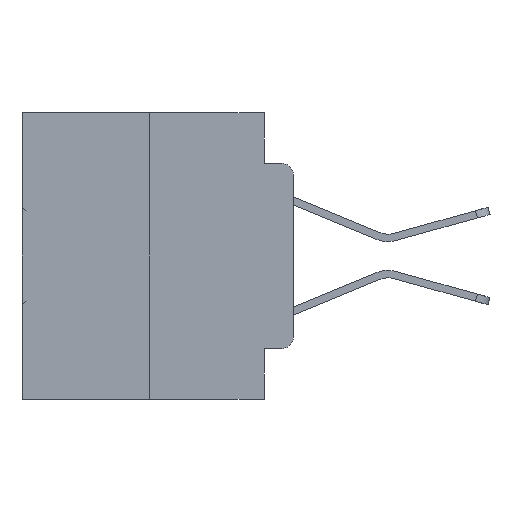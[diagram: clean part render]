
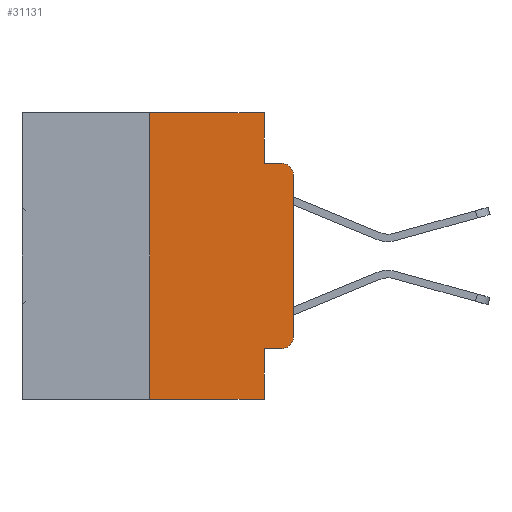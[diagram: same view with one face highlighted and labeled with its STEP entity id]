
A CAD part, left-side view. The second image highlights one B-rep face of the part: STEP entity #31131.
In plain terms, the highlighted planar face has unit normal (-1, 0, 0).
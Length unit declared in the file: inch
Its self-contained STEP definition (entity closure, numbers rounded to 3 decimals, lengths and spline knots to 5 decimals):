
#1025 = ORIENTED_EDGE ( 'NONE', *, *, #8516, .F. ) ;
#1238 = VERTEX_POINT ( 'NONE', #7258 ) ;
#1421 = ORIENTED_EDGE ( 'NONE', *, *, #26713, .T. ) ;
#1630 = EDGE_CURVE ( 'NONE', #18793, #30421, #24792, .T. ) ;
#1648 = VERTEX_POINT ( 'NONE', #25018 ) ;
#1846 = ORIENTED_EDGE ( 'NONE', *, *, #18257, .T. ) ;
#1852 = CARTESIAN_POINT ( 'NONE',  ( 0., 0.473, -0.5 ) ) ;
#3030 = ORIENTED_EDGE ( 'NONE', *, *, #29898, .F. ) ;
#3346 = EDGE_CURVE ( 'NONE', #16393, #30421, #4050, .T. ) ;
#3467 = DIRECTION ( 'NONE',  ( 0., 0., 1. ) ) ;
#3589 = CARTESIAN_POINT ( 'NONE',  ( 0., 0.051, -0.4115 ) ) ;
#3767 = VECTOR ( 'NONE', #28700, 39.37008 ) ;
#3779 = CARTESIAN_POINT ( 'NONE',  ( 0., 0.25, -0.5 ) ) ;
#4050 = LINE ( 'NONE', #28193, #22817 ) ;
#4171 = CARTESIAN_POINT ( 'NONE',  ( 0., 0.473, 0. ) ) ;
#4619 = VERTEX_POINT ( 'NONE', #8274 ) ;
#4640 = ORIENTED_EDGE ( 'NONE', *, *, #25094, .F. ) ;
#4883 = AXIS2_PLACEMENT_3D ( 'NONE', #17236, #7419, #24492 ) ;
#4959 = PLANE ( 'NONE',  #4883 ) ;
#5057 = LINE ( 'NONE', #21736, #17384 ) ;
#5177 = DIRECTION ( 'NONE',  ( 0., 0., -1. ) ) ;
#5920 = LINE ( 'NONE', #28124, #19065 ) ;
#7258 = CARTESIAN_POINT ( 'NONE',  ( 0., 0., -0.3915 ) ) ;
#7419 = DIRECTION ( 'NONE',  ( 1., 0., 0. ) ) ;
#7840 = LINE ( 'NONE', #20682, #15943 ) ;
#8078 = ORIENTED_EDGE ( 'NONE', *, *, #1630, .T. ) ;
#8274 = CARTESIAN_POINT ( 'NONE',  ( 0., 0.02, -0.4115 ) ) ;
#8516 = EDGE_CURVE ( 'NONE', #19788, #1648, #23984, .T. ) ;
#9701 = EDGE_LOOP ( 'NONE', ( #1421, #8078, #21119, #3030, #16188, #4640, #12731, #1025, #14278, #1846 ) ) ;
#9738 = CARTESIAN_POINT ( 'NONE',  ( 0., 0.051, -0.4115 ) ) ;
#10008 = CIRCLE ( 'NONE', #16569, 0.02 ) ;
#11039 = VECTOR ( 'NONE', #5177, 39.37008 ) ;
#11698 = AXIS2_PLACEMENT_3D ( 'NONE', #22172, #13034, #18883 ) ;
#12731 = ORIENTED_EDGE ( 'NONE', *, *, #18904, .T. ) ;
#13034 = DIRECTION ( 'NONE',  ( -1., 0., 0. ) ) ;
#13632 = DIRECTION ( 'NONE',  ( 0., 0., -1. ) ) ;
#13913 = CARTESIAN_POINT ( 'NONE',  ( 0., 0., -0.1085 ) ) ;
#14278 = ORIENTED_EDGE ( 'NONE', *, *, #18343, .T. ) ;
#14365 = CARTESIAN_POINT ( 'NONE',  ( 0., 0.051, -0.0885 ) ) ;
#14369 = DIRECTION ( 'NONE',  ( -1., 0., 0. ) ) ;
#15943 = VECTOR ( 'NONE', #3467, 39.37008 ) ;
#16188 = ORIENTED_EDGE ( 'NONE', *, *, #26628, .F. ) ;
#16339 = VERTEX_POINT ( 'NONE', #28628 ) ;
#16393 = VERTEX_POINT ( 'NONE', #14365 ) ;
#16569 = AXIS2_PLACEMENT_3D ( 'NONE', #28843, #14369, #31193 ) ;
#17058 = DIRECTION ( 'NONE',  ( 0., -1., 0. ) ) ;
#17236 = CARTESIAN_POINT ( 'NONE',  ( 0., 0.473, 0. ) ) ;
#17384 = VECTOR ( 'NONE', #24153, 39.37008 ) ;
#18257 = EDGE_CURVE ( 'NONE', #4619, #1238, #10008, .T. ) ;
#18343 = EDGE_CURVE ( 'NONE', #19788, #4619, #26346, .T. ) ;
#18793 = VERTEX_POINT ( 'NONE', #13913 ) ;
#18883 = DIRECTION ( 'NONE',  ( 0., 0., -1. ) ) ;
#18904 = EDGE_CURVE ( 'NONE', #27709, #1648, #29679, .T. ) ;
#19065 = VECTOR ( 'NONE', #13632, 39.37008 ) ;
#19788 = VERTEX_POINT ( 'NONE', #3589 ) ;
#19915 = CARTESIAN_POINT ( 'NONE',  ( 0., 0.051, 0. ) ) ;
#20430 = LINE ( 'NONE', #4171, #26042 ) ;
#20534 = CARTESIAN_POINT ( 'NONE',  ( 0., 0.02, -0.0885 ) ) ;
#20682 = CARTESIAN_POINT ( 'NONE',  ( 0., 0.25, 0. ) ) ;
#21119 = ORIENTED_EDGE ( 'NONE', *, *, #3346, .F. ) ;
#21420 = DIRECTION ( 'NONE',  ( 0., -1., 0. ) ) ;
#21736 = CARTESIAN_POINT ( 'NONE',  ( 0., 0., 0. ) ) ;
#22172 = CARTESIAN_POINT ( 'NONE',  ( 0., 0.02, -0.1085 ) ) ;
#22331 = DIRECTION ( 'NONE',  ( 0., -1., 0. ) ) ;
#22817 = VECTOR ( 'NONE', #22331, 39.37008 ) ;
#23984 = LINE ( 'NONE', #19915, #11039 ) ;
#24153 = DIRECTION ( 'NONE',  ( 0., 0., 1. ) ) ;
#24492 = DIRECTION ( 'NONE',  ( 0., 0., -1. ) ) ;
#24792 = CIRCLE ( 'NONE', #11698, 0.02 ) ;
#25018 = CARTESIAN_POINT ( 'NONE',  ( 0., 0.051, -0.5 ) ) ;
#25094 = EDGE_CURVE ( 'NONE', #27709, #31348, #7840, .T. ) ;
#25593 = VECTOR ( 'NONE', #17058, 39.37008 ) ;
#25751 = FACE_OUTER_BOUND ( 'NONE', #9701, .T. ) ;
#26042 = VECTOR ( 'NONE', #21420, 39.37008 ) ;
#26346 = LINE ( 'NONE', #9738, #25593 ) ;
#26628 = EDGE_CURVE ( 'NONE', #31348, #16339, #20430, .T. ) ;
#26713 = EDGE_CURVE ( 'NONE', #1238, #18793, #5057, .T. ) ;
#27709 = VERTEX_POINT ( 'NONE', #3779 ) ;
#28124 = CARTESIAN_POINT ( 'NONE',  ( 0., 0.051, 0. ) ) ;
#28193 = CARTESIAN_POINT ( 'NONE',  ( 0., 0.051, -0.0885 ) ) ;
#28628 = CARTESIAN_POINT ( 'NONE',  ( 0., 0.051, 0. ) ) ;
#28700 = DIRECTION ( 'NONE',  ( 0., -1., 0. ) ) ;
#28843 = CARTESIAN_POINT ( 'NONE',  ( 0., 0.02, -0.3915 ) ) ;
#29679 = LINE ( 'NONE', #1852, #3767 ) ;
#29898 = EDGE_CURVE ( 'NONE', #16339, #16393, #5920, .T. ) ;
#30125 = CARTESIAN_POINT ( 'NONE',  ( 0., 0.25, 0. ) ) ;
#30421 = VERTEX_POINT ( 'NONE', #20534 ) ;
#31131 = ADVANCED_FACE ( 'NONE', ( #25751 ), #4959, .F. ) ;
#31193 = DIRECTION ( 'NONE',  ( 0., 0., -1. ) ) ;
#31348 = VERTEX_POINT ( 'NONE', #30125 ) ;
